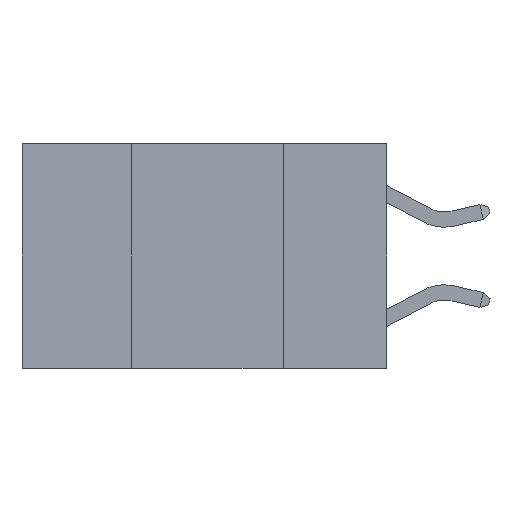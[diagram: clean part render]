
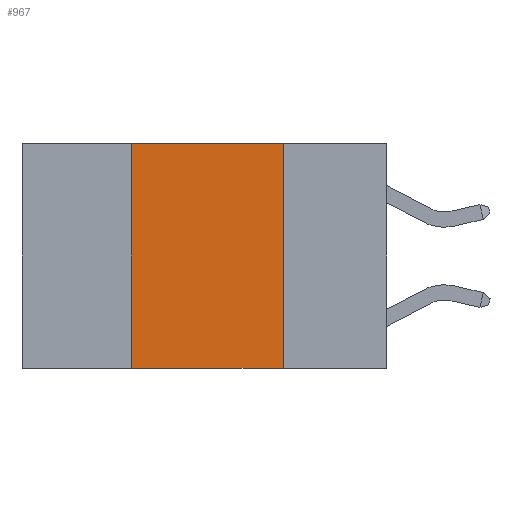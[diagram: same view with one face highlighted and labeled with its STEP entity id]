
A CAD part, left-side view. The second image highlights one B-rep face of the part: STEP entity #967.
In plain terms, the highlighted planar face has unit normal (-1, 0, 0).
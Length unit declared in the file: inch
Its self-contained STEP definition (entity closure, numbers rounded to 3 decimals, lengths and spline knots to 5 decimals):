
#69 = DIRECTION ( 'NONE',  ( 0., -1., 0. ) ) ;
#652 = LINE ( 'NONE', #6348, #24734 ) ;
#967 = ADVANCED_FACE ( 'NONE', ( #29139 ), #4614, .F. ) ;
#1126 = DIRECTION ( 'NONE',  ( 1., 0., 0. ) ) ;
#2898 = EDGE_LOOP ( 'NONE', ( #8843, #20910, #4236, #16321 ) ) ;
#3681 = VECTOR ( 'NONE', #18213, 39.37008 ) ;
#4236 = ORIENTED_EDGE ( 'NONE', *, *, #26511, .F. ) ;
#4614 = PLANE ( 'NONE',  #14736 ) ;
#6348 = CARTESIAN_POINT ( 'NONE',  ( 0., 0.17, 0. ) ) ;
#8843 = ORIENTED_EDGE ( 'NONE', *, *, #24764, .F. ) ;
#9245 = CARTESIAN_POINT ( 'NONE',  ( 0., 0.6, 0. ) ) ;
#9851 = VERTEX_POINT ( 'NONE', #26518 ) ;
#10161 = LINE ( 'NONE', #12807, #27572 ) ;
#12684 = DIRECTION ( 'NONE',  ( 0., 0., -1. ) ) ;
#12807 = CARTESIAN_POINT ( 'NONE',  ( 0., 0.6, 0. ) ) ;
#13626 = CARTESIAN_POINT ( 'NONE',  ( 0., 0.42, 0. ) ) ;
#14736 = AXIS2_PLACEMENT_3D ( 'NONE', #9245, #1126, #12684 ) ;
#16321 = ORIENTED_EDGE ( 'NONE', *, *, #19811, .T. ) ;
#17892 = CARTESIAN_POINT ( 'NONE',  ( 0., 0.42, 0. ) ) ;
#17953 = CARTESIAN_POINT ( 'NONE',  ( 0., 0.17, -0.37 ) ) ;
#18213 = DIRECTION ( 'NONE',  ( 0., 0., 1. ) ) ;
#19393 = CARTESIAN_POINT ( 'NONE',  ( 0., 0.42, -0.37 ) ) ;
#19811 = EDGE_CURVE ( 'NONE', #21427, #20998, #26520, .T. ) ;
#20292 = VERTEX_POINT ( 'NONE', #17892 ) ;
#20474 = VECTOR ( 'NONE', #69, 39.37008 ) ;
#20910 = ORIENTED_EDGE ( 'NONE', *, *, #25534, .F. ) ;
#20998 = VERTEX_POINT ( 'NONE', #17953 ) ;
#21427 = VERTEX_POINT ( 'NONE', #19393 ) ;
#21736 = LINE ( 'NONE', #13626, #3681 ) ;
#22148 = DIRECTION ( 'NONE',  ( 0., 0., -1. ) ) ;
#24734 = VECTOR ( 'NONE', #22148, 39.37008 ) ;
#24764 = EDGE_CURVE ( 'NONE', #9851, #20998, #652, .T. ) ;
#24912 = CARTESIAN_POINT ( 'NONE',  ( 0., 0.6, -0.37 ) ) ;
#25534 = EDGE_CURVE ( 'NONE', #20292, #9851, #10161, .T. ) ;
#26390 = DIRECTION ( 'NONE',  ( 0., -1., 0. ) ) ;
#26511 = EDGE_CURVE ( 'NONE', #21427, #20292, #21736, .T. ) ;
#26518 = CARTESIAN_POINT ( 'NONE',  ( 0., 0.17, 0. ) ) ;
#26520 = LINE ( 'NONE', #24912, #20474 ) ;
#27572 = VECTOR ( 'NONE', #26390, 39.37008 ) ;
#29139 = FACE_OUTER_BOUND ( 'NONE', #2898, .T. ) ;
